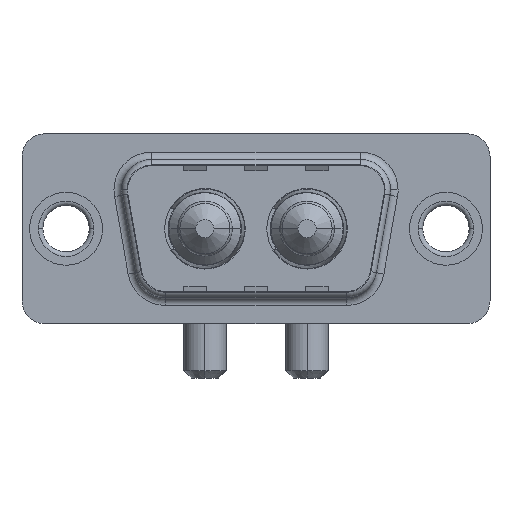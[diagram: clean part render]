
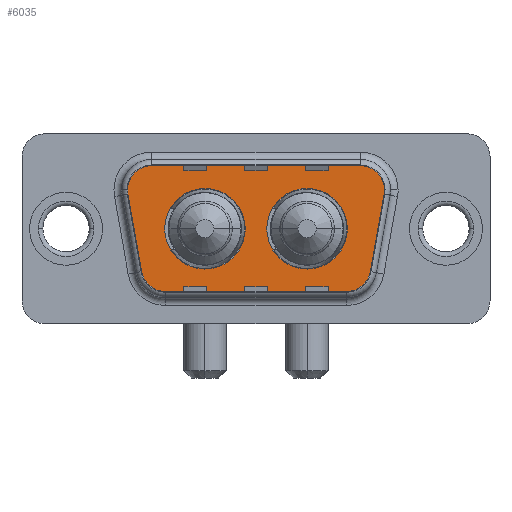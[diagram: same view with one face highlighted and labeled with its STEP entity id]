
A CAD part, top view. The second image highlights one B-rep face of the part: STEP entity #6035.
In plain terms, the highlighted planar face has unit normal (0, 0, 1).
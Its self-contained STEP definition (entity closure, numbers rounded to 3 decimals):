
#14 = EDGE_CURVE ( 'NONE', #3590, #5815, #7868, .T. ) ;
#22 = AXIS2_PLACEMENT_3D ( 'NONE', #6049, #3176, #9095 ) ;
#53 = DIRECTION ( 'NONE',  ( 1., 0., 0. ) ) ;
#159 = DIRECTION ( 'NONE',  ( 0., 0., 1. ) ) ;
#165 = DIRECTION ( 'NONE',  ( 0., 0., 1. ) ) ;
#236 = VERTEX_POINT ( 'NONE', #5993 ) ;
#276 = ORIENTED_EDGE ( 'NONE', *, *, #2215, .T. ) ;
#346 = VERTEX_POINT ( 'NONE', #1778 ) ;
#401 = DIRECTION ( 'NONE',  ( 0., 0., 1. ) ) ;
#429 = ORIENTED_EDGE ( 'NONE', *, *, #6828, .T. ) ;
#445 = ORIENTED_EDGE ( 'NONE', *, *, #728, .T. ) ;
#460 = ORIENTED_EDGE ( 'NONE', *, *, #3556, .T. ) ;
#499 = CIRCLE ( 'NONE', #6658, 2. ) ;
#542 = DIRECTION ( 'NONE',  ( -1., 0., 0. ) ) ;
#579 = FACE_OUTER_BOUND ( 'NONE', #3178, .T. ) ;
#608 = EDGE_CURVE ( 'NONE', #1004, #4919, #5837, .T. ) ;
#632 = DIRECTION ( 'NONE',  ( 0.174, 0.985, 0. ) ) ;
#644 = CIRCLE ( 'NONE', #22, 2.65 ) ;
#728 = EDGE_CURVE ( 'NONE', #346, #2344, #2358, .T. ) ;
#740 = CARTESIAN_POINT ( 'NONE',  ( 6.459, -2.9, 0. ) ) ;
#922 = ORIENTED_EDGE ( 'NONE', *, *, #608, .F. ) ;
#1004 = VERTEX_POINT ( 'NONE', #4069 ) ;
#1163 = VERTEX_POINT ( 'NONE', #2179 ) ;
#1274 = CARTESIAN_POINT ( 'NONE',  ( 21.534, 2.553, 0. ) ) ;
#1331 = DIRECTION ( 'NONE',  ( 0., 0., 1. ) ) ;
#1433 = EDGE_CURVE ( 'NONE', #5904, #5194, #499, .T. ) ;
#1560 = CARTESIAN_POINT ( 'NONE',  ( 4.489, -3.247, 0. ) ) ;
#1610 = DIRECTION ( 'NONE',  ( 1., 0., 0. ) ) ;
#1778 = CARTESIAN_POINT ( 'NONE',  ( 18.541, -4.9, 0. ) ) ;
#1842 = AXIS2_PLACEMENT_3D ( 'NONE', #6930, #159, #6838 ) ;
#1845 = EDGE_LOOP ( 'NONE', ( #7249, #3322 ) ) ;
#1947 = LINE ( 'NONE', #3339, #3336 ) ;
#2013 = CARTESIAN_POINT ( 'NONE',  ( 18.541, -2.9, 0. ) ) ;
#2036 = AXIS2_PLACEMENT_3D ( 'NONE', #3276, #165, #8003 ) ;
#2179 = CARTESIAN_POINT ( 'NONE',  ( 18.51, 0., 0. ) ) ;
#2215 = EDGE_CURVE ( 'NONE', #5567, #3590, #5449, .T. ) ;
#2218 = CARTESIAN_POINT ( 'NONE',  ( 21.564, 2.9, 0. ) ) ;
#2235 = ORIENTED_EDGE ( 'NONE', *, *, #7191, .T. ) ;
#2299 = EDGE_CURVE ( 'NONE', #236, #346, #4122, .T. ) ;
#2344 = VERTEX_POINT ( 'NONE', #8951 ) ;
#2358 = CIRCLE ( 'NONE', #6313, 2. ) ;
#2440 = EDGE_LOOP ( 'NONE', ( #922, #4237 ) ) ;
#2468 = ORIENTED_EDGE ( 'NONE', *, *, #5684, .T. ) ;
#2476 = EDGE_CURVE ( 'NONE', #3317, #1163, #9732, .T. ) ;
#2662 = ORIENTED_EDGE ( 'NONE', *, *, #14, .T. ) ;
#2713 = VECTOR ( 'NONE', #632, 1000. ) ;
#3057 = DIRECTION ( 'NONE',  ( 0., 0., 1. ) ) ;
#3090 = VECTOR ( 'NONE', #6216, 1000. ) ;
#3176 = DIRECTION ( 'NONE',  ( 0., 0., 1. ) ) ;
#3178 = EDGE_LOOP ( 'NONE', ( #445, #2468, #4812, #2235, #460, #276, #2662, #429, #4246 ) ) ;
#3276 = CARTESIAN_POINT ( 'NONE',  ( 9.14, 0., 0. ) ) ;
#3284 = DIRECTION ( 'NONE',  ( 0., 0., 1. ) ) ;
#3317 = VERTEX_POINT ( 'NONE', #6671 ) ;
#3322 = ORIENTED_EDGE ( 'NONE', *, *, #2476, .F. ) ;
#3336 = VECTOR ( 'NONE', #6459, 1000. ) ;
#3339 = CARTESIAN_POINT ( 'NONE',  ( 5.436, 4.9, 0. ) ) ;
#3371 = CIRCLE ( 'NONE', #8430, 2. ) ;
#3440 = VECTOR ( 'NONE', #7276, 1000. ) ;
#3487 = PLANE ( 'NONE',  #3675 ) ;
#3556 = EDGE_CURVE ( 'NONE', #9314, #5567, #1947, .T. ) ;
#3588 = FACE_BOUND ( 'NONE', #1845, .T. ) ;
#3590 = VERTEX_POINT ( 'NONE', #5963 ) ;
#3675 = AXIS2_PLACEMENT_3D ( 'NONE', #8777, #4280, #9613 ) ;
#3879 = AXIS2_PLACEMENT_3D ( 'NONE', #6502, #4726, #1610 ) ;
#4042 = CARTESIAN_POINT ( 'NONE',  ( 21.534, 2.553, 0. ) ) ;
#4069 = CARTESIAN_POINT ( 'NONE',  ( 11.79, 0., 0. ) ) ;
#4122 = LINE ( 'NONE', #7696, #3090 ) ;
#4237 = ORIENTED_EDGE ( 'NONE', *, *, #4585, .F. ) ;
#4246 = ORIENTED_EDGE ( 'NONE', *, *, #2299, .T. ) ;
#4280 = DIRECTION ( 'NONE',  ( 0., 0., 1. ) ) ;
#4345 = EDGE_CURVE ( 'NONE', #1163, #3317, #644, .T. ) ;
#4404 = CARTESIAN_POINT ( 'NONE',  ( 6.49, 0., 0. ) ) ;
#4585 = EDGE_CURVE ( 'NONE', #4919, #1004, #5683, .T. ) ;
#4726 = DIRECTION ( 'NONE',  ( 0., 0., 1. ) ) ;
#4812 = ORIENTED_EDGE ( 'NONE', *, *, #1433, .T. ) ;
#4919 = VERTEX_POINT ( 'NONE', #4404 ) ;
#4977 = FACE_BOUND ( 'NONE', #2440, .T. ) ;
#5194 = VERTEX_POINT ( 'NONE', #2218 ) ;
#5449 = CIRCLE ( 'NONE', #3879, 2. ) ;
#5462 = CARTESIAN_POINT ( 'NONE',  ( 19.564, 2.9, 0. ) ) ;
#5562 = DIRECTION ( 'NONE',  ( -1., 0., 0. ) ) ;
#5567 = VERTEX_POINT ( 'NONE', #9379 ) ;
#5660 = CARTESIAN_POINT ( 'NONE',  ( 19.564, 4.9, 0. ) ) ;
#5683 = CIRCLE ( 'NONE', #2036, 2.65 ) ;
#5684 = EDGE_CURVE ( 'NONE', #2344, #5904, #9670, .T. ) ;
#5815 = VERTEX_POINT ( 'NONE', #1560 ) ;
#5837 = CIRCLE ( 'NONE', #9621, 2.65 ) ;
#5904 = VERTEX_POINT ( 'NONE', #4042 ) ;
#5963 = CARTESIAN_POINT ( 'NONE',  ( 3.466, 2.553, 0. ) ) ;
#5993 = CARTESIAN_POINT ( 'NONE',  ( 6.459, -4.9, 0. ) ) ;
#6035 = ADVANCED_FACE ( 'NONE', ( #3588, #4977, #579 ), #3487, .T. ) ;
#6049 = CARTESIAN_POINT ( 'NONE',  ( 15.86, 0., 0. ) ) ;
#6216 = DIRECTION ( 'NONE',  ( 1., 0., 0. ) ) ;
#6313 = AXIS2_PLACEMENT_3D ( 'NONE', #2013, #3057, #53 ) ;
#6375 = AXIS2_PLACEMENT_3D ( 'NONE', #740, #6529, #542 ) ;
#6434 = DIRECTION ( 'NONE',  ( -1., 0., 0. ) ) ;
#6459 = DIRECTION ( 'NONE',  ( -1., 0., 0. ) ) ;
#6495 = CARTESIAN_POINT ( 'NONE',  ( 3.466, 2.553, 0. ) ) ;
#6502 = CARTESIAN_POINT ( 'NONE',  ( 5.436, 2.9, 0. ) ) ;
#6529 = DIRECTION ( 'NONE',  ( 0., 0., 1. ) ) ;
#6658 = AXIS2_PLACEMENT_3D ( 'NONE', #7170, #401, #6434 ) ;
#6671 = CARTESIAN_POINT ( 'NONE',  ( 13.21, 0., 0. ) ) ;
#6828 = EDGE_CURVE ( 'NONE', #5815, #236, #7630, .T. ) ;
#6838 = DIRECTION ( 'NONE',  ( 1., 0., 0. ) ) ;
#6930 = CARTESIAN_POINT ( 'NONE',  ( 15.86, 0., 0. ) ) ;
#7170 = CARTESIAN_POINT ( 'NONE',  ( 19.564, 2.9, 0. ) ) ;
#7191 = EDGE_CURVE ( 'NONE', #5194, #9314, #3371, .T. ) ;
#7249 = ORIENTED_EDGE ( 'NONE', *, *, #4345, .F. ) ;
#7276 = DIRECTION ( 'NONE',  ( 0.174, -0.985, 0. ) ) ;
#7630 = CIRCLE ( 'NONE', #6375, 2. ) ;
#7696 = CARTESIAN_POINT ( 'NONE',  ( 6.459, -4.9, 0. ) ) ;
#7868 = LINE ( 'NONE', #6495, #3440 ) ;
#8003 = DIRECTION ( 'NONE',  ( 1., 0., 0. ) ) ;
#8430 = AXIS2_PLACEMENT_3D ( 'NONE', #5462, #3284, #5562 ) ;
#8777 = CARTESIAN_POINT ( 'NONE',  ( 18.541, -2.9, 0. ) ) ;
#8839 = DIRECTION ( 'NONE',  ( 1., 0., 0. ) ) ;
#8951 = CARTESIAN_POINT ( 'NONE',  ( 20.511, -3.247, 0. ) ) ;
#9095 = DIRECTION ( 'NONE',  ( 1., 0., 0. ) ) ;
#9314 = VERTEX_POINT ( 'NONE', #5660 ) ;
#9379 = CARTESIAN_POINT ( 'NONE',  ( 5.436, 4.9, 0. ) ) ;
#9613 = DIRECTION ( 'NONE',  ( 1., 0., 0. ) ) ;
#9621 = AXIS2_PLACEMENT_3D ( 'NONE', #9676, #1331, #8839 ) ;
#9670 = LINE ( 'NONE', #1274, #2713 ) ;
#9676 = CARTESIAN_POINT ( 'NONE',  ( 9.14, 0., 0. ) ) ;
#9732 = CIRCLE ( 'NONE', #1842, 2.65 ) ;
